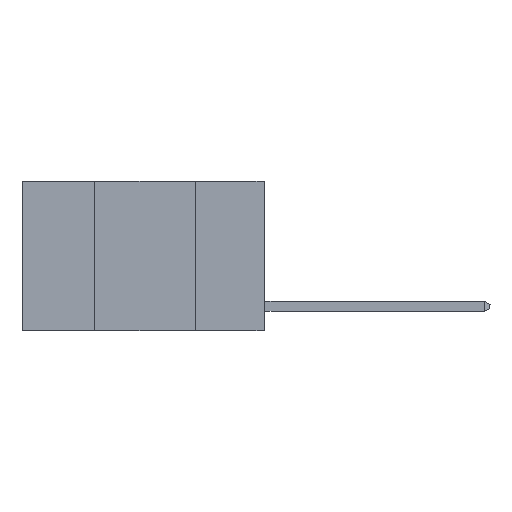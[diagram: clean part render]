
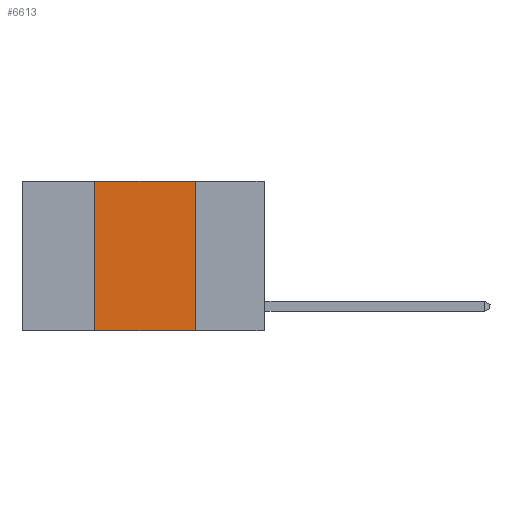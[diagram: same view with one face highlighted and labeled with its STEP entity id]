
A CAD part, left-side view. The second image highlights one B-rep face of the part: STEP entity #6613.
In plain terms, the highlighted planar face has unit normal (-1, 0, 0).
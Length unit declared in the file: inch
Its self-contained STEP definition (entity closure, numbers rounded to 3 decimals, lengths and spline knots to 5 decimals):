
#592 = EDGE_CURVE ( 'NONE', #4924, #15065, #21926, .T. ) ;
#1176 = FACE_OUTER_BOUND ( 'NONE', #14265, .T. ) ;
#1244 = CARTESIAN_POINT ( 'NONE',  ( 0., 0.6, 0. ) ) ;
#1868 = LINE ( 'NONE', #5719, #25537 ) ;
#2085 = DIRECTION ( 'NONE',  ( 0., 0., -1. ) ) ;
#2345 = DIRECTION ( 'NONE',  ( 0., 0., 1. ) ) ;
#3111 = LINE ( 'NONE', #6983, #3827 ) ;
#3215 = ORIENTED_EDGE ( 'NONE', *, *, #12652, .T. ) ;
#3532 = CARTESIAN_POINT ( 'NONE',  ( 0., 0.17, -0.37 ) ) ;
#3579 = VECTOR ( 'NONE', #9457, 39.37008 ) ;
#3827 = VECTOR ( 'NONE', #2345, 39.37008 ) ;
#4924 = VERTEX_POINT ( 'NONE', #23647 ) ;
#5719 = CARTESIAN_POINT ( 'NONE',  ( 0., 0.6, -0.37 ) ) ;
#5760 = CARTESIAN_POINT ( 'NONE',  ( 0., 0.42, -0.37 ) ) ;
#6109 = PLANE ( 'NONE',  #6479 ) ;
#6479 = AXIS2_PLACEMENT_3D ( 'NONE', #22178, #8455, #24450 ) ;
#6613 = ADVANCED_FACE ( 'NONE', ( #1176 ), #6109, .F. ) ;
#6983 = CARTESIAN_POINT ( 'NONE',  ( 0., 0.42, 0. ) ) ;
#8455 = DIRECTION ( 'NONE',  ( 1., 0., 0. ) ) ;
#9457 = DIRECTION ( 'NONE',  ( 0., -1., 0. ) ) ;
#10065 = EDGE_CURVE ( 'NONE', #16182, #4924, #3111, .T. ) ;
#12652 = EDGE_CURVE ( 'NONE', #16182, #25665, #1868, .T. ) ;
#14265 = EDGE_LOOP ( 'NONE', ( #15709, #14715, #23654, #3215 ) ) ;
#14288 = LINE ( 'NONE', #15922, #25681 ) ;
#14715 = ORIENTED_EDGE ( 'NONE', *, *, #592, .F. ) ;
#15065 = VERTEX_POINT ( 'NONE', #29308 ) ;
#15709 = ORIENTED_EDGE ( 'NONE', *, *, #24601, .F. ) ;
#15922 = CARTESIAN_POINT ( 'NONE',  ( 0., 0.17, 0. ) ) ;
#16182 = VERTEX_POINT ( 'NONE', #5760 ) ;
#21926 = LINE ( 'NONE', #1244, #3579 ) ;
#22178 = CARTESIAN_POINT ( 'NONE',  ( 0., 0.6, 0. ) ) ;
#23647 = CARTESIAN_POINT ( 'NONE',  ( 0., 0.42, 0. ) ) ;
#23654 = ORIENTED_EDGE ( 'NONE', *, *, #10065, .F. ) ;
#24450 = DIRECTION ( 'NONE',  ( 0., 0., -1. ) ) ;
#24601 = EDGE_CURVE ( 'NONE', #15065, #25665, #14288, .T. ) ;
#25537 = VECTOR ( 'NONE', #26345, 39.37008 ) ;
#25665 = VERTEX_POINT ( 'NONE', #3532 ) ;
#25681 = VECTOR ( 'NONE', #2085, 39.37008 ) ;
#26345 = DIRECTION ( 'NONE',  ( 0., -1., 0. ) ) ;
#29308 = CARTESIAN_POINT ( 'NONE',  ( 0., 0.17, 0. ) ) ;
